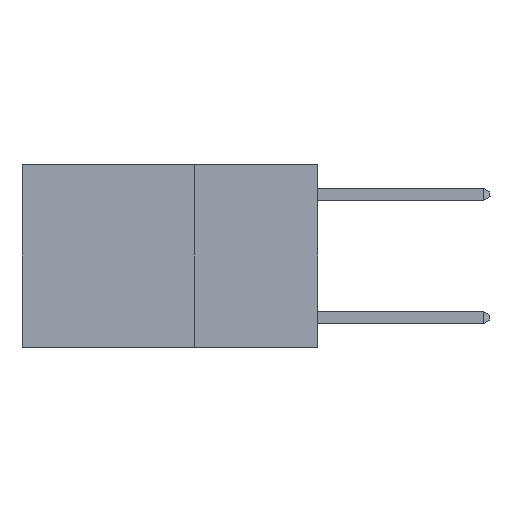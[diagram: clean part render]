
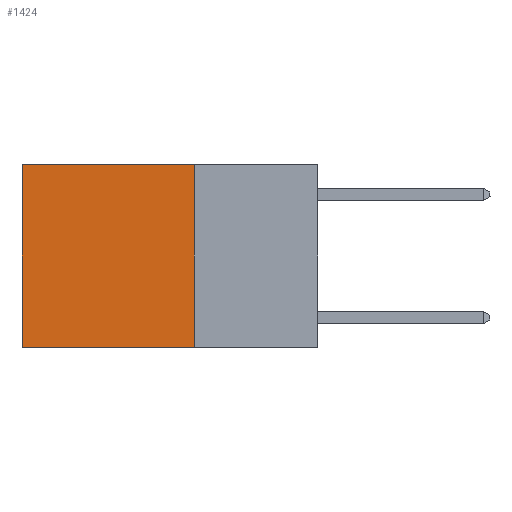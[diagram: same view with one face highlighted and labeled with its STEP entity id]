
A CAD part, left-side view. The second image highlights one B-rep face of the part: STEP entity #1424.
In plain terms, the highlighted planar face has unit normal (-1, 0, 0).
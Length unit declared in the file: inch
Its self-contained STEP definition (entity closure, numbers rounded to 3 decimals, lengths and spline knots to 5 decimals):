
#208 = CARTESIAN_POINT ( 'NONE',  ( 0.2625, 0.6, 0. ) ) ;
#524 = DIRECTION ( 'NONE',  ( 0., 1., 0. ) ) ;
#610 = EDGE_CURVE ( 'NONE', #1556, #891, #3960, .T. ) ;
#627 = LINE ( 'NONE', #4548, #3036 ) ;
#891 = VERTEX_POINT ( 'NONE', #5173 ) ;
#1337 = EDGE_CURVE ( 'NONE', #6631, #8127, #11119, .T. ) ;
#1424 = ADVANCED_FACE ( 'NONE', ( #9478 ), #6498, .F. ) ;
#1556 = VERTEX_POINT ( 'NONE', #5061 ) ;
#1873 = DIRECTION ( 'NONE',  ( 1., 0., 0. ) ) ;
#2092 = ORIENTED_EDGE ( 'NONE', *, *, #2757, .F. ) ;
#2346 = DIRECTION ( 'NONE',  ( 0., 0., -1. ) ) ;
#2704 = ORIENTED_EDGE ( 'NONE', *, *, #610, .T. ) ;
#2757 = EDGE_CURVE ( 'NONE', #1556, #6631, #627, .T. ) ;
#2784 = CARTESIAN_POINT ( 'NONE',  ( 0.2625, 0.25, -0.37 ) ) ;
#3036 = VECTOR ( 'NONE', #9987, 39.37008 ) ;
#3664 = AXIS2_PLACEMENT_3D ( 'NONE', #10975, #1873, #8332 ) ;
#3694 = LINE ( 'NONE', #208, #8243 ) ;
#3929 = VECTOR ( 'NONE', #524, 39.37008 ) ;
#3960 = LINE ( 'NONE', #9921, #11145 ) ;
#4014 = ORIENTED_EDGE ( 'NONE', *, *, #11835, .T. ) ;
#4157 = CARTESIAN_POINT ( 'NONE',  ( 0.2625, 0.6, -0.37 ) ) ;
#4482 = DIRECTION ( 'NONE',  ( 0., 1., 0. ) ) ;
#4548 = CARTESIAN_POINT ( 'NONE',  ( 0.2625, 0.25, 0. ) ) ;
#5061 = CARTESIAN_POINT ( 'NONE',  ( 0.2625, 0.25, 0. ) ) ;
#5173 = CARTESIAN_POINT ( 'NONE',  ( 0.2625, 0.6, 0. ) ) ;
#6498 = PLANE ( 'NONE',  #3664 ) ;
#6631 = VERTEX_POINT ( 'NONE', #2784 ) ;
#8103 = CARTESIAN_POINT ( 'NONE',  ( 0.2625, 0.25, -0.37 ) ) ;
#8127 = VERTEX_POINT ( 'NONE', #4157 ) ;
#8243 = VECTOR ( 'NONE', #2346, 39.37008 ) ;
#8332 = DIRECTION ( 'NONE',  ( 0., 0., -1. ) ) ;
#8859 = ORIENTED_EDGE ( 'NONE', *, *, #1337, .F. ) ;
#8900 = EDGE_LOOP ( 'NONE', ( #4014, #8859, #2092, #2704 ) ) ;
#9478 = FACE_OUTER_BOUND ( 'NONE', #8900, .T. ) ;
#9921 = CARTESIAN_POINT ( 'NONE',  ( 0.2625, 0.25, 0. ) ) ;
#9987 = DIRECTION ( 'NONE',  ( 0., 0., -1. ) ) ;
#10975 = CARTESIAN_POINT ( 'NONE',  ( 0.2625, 0.25, 0. ) ) ;
#11119 = LINE ( 'NONE', #8103, #3929 ) ;
#11145 = VECTOR ( 'NONE', #4482, 39.37008 ) ;
#11835 = EDGE_CURVE ( 'NONE', #891, #8127, #3694, .T. ) ;
